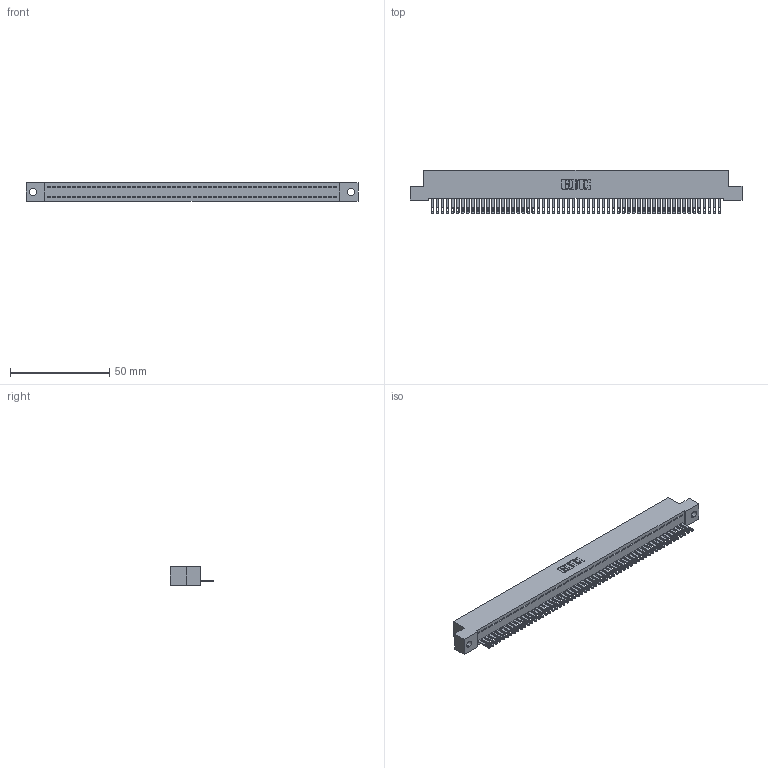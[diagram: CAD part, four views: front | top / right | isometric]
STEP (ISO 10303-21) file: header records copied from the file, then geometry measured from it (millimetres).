
FILE_DESCRIPTION (( 'STEP AP203' ), '1' );
FILE_NAME ('342-058-500-102.STEP', '2019-10-03T12:17:11', ( '' ), ( '' ), 'SwSTEP 2.0', 'SolidWorks 2016', '' );
FILE_SCHEMA (( 'CONFIG_CONTROL_DESIGN' ));
Length unit declared in the file: inch
Products named in the file (3): 342 Part_.128 Slot; 345-292-001_345-293-100; 342-058-500-102
Assembly tree (59 placements, depth 2):
  342-058-500-102
    342 Part_.128 Slot
    345-292-001_345-293-100  x58
Bounding box: 167.64 x 21.85 x 9.4 mm (x, y, z)
Volume: 14741.4 mm3; surface area: 21819.6 mm2
Topology: 59 solids, 59 shells, 3246 faces, 10055 edges, 6702 vertices
Faces by surface type: plane 2158, cylinder 1088
Entity records: 33321 total; most frequent: CARTESIAN_POINT 5752, ORIENTED_EDGE 5746, DIRECTION 4821, EDGE_CURVE 2873, VECTOR 2741, LINE 2741, VERTEX_POINT 1914, AXIS2_PLACEMENT_3D 1040
